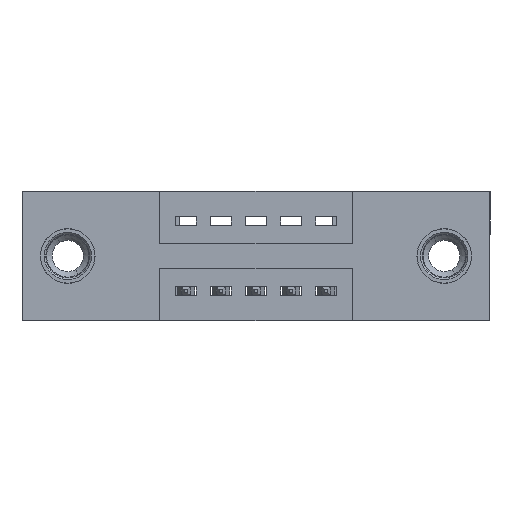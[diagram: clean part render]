
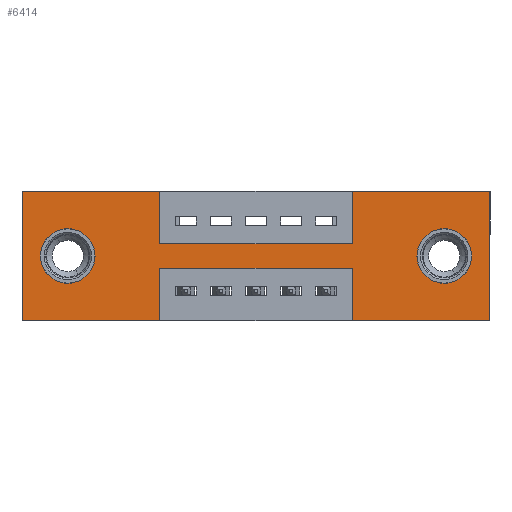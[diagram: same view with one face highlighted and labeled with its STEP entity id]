
A CAD part, front view. The second image highlights one B-rep face of the part: STEP entity #6414.
In plain terms, the highlighted planar face has unit normal (0, -1, 0).
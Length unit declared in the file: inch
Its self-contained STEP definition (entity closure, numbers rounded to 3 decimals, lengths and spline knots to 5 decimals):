
#1 = EDGE_CURVE ( 'NONE', #5231, #4757, #5627, .T. ) ;
#156 = CARTESIAN_POINT ( 'NONE',  ( 1.335, 0., 0. ) ) ;
#190 = VECTOR ( 'NONE', #808, 39.37008 ) ;
#221 = DIRECTION ( 'NONE',  ( 1., 0., 0. ) ) ;
#294 = ORIENTED_EDGE ( 'NONE', *, *, #10173, .F. ) ;
#348 = DIRECTION ( 'NONE',  ( 0., 0., -1. ) ) ;
#634 = CARTESIAN_POINT ( 'NONE',  ( 0.9425, 0., -0.37 ) ) ;
#799 = ORIENTED_EDGE ( 'NONE', *, *, #4436, .T. ) ;
#808 = DIRECTION ( 'NONE',  ( -1., 0., 0. ) ) ;
#852 = DIRECTION ( 'NONE',  ( 1., 0., 0. ) ) ;
#879 = VECTOR ( 'NONE', #11801, 39.37008 ) ;
#882 = VERTEX_POINT ( 'NONE', #13210 ) ;
#1131 = ORIENTED_EDGE ( 'NONE', *, *, #8458, .F. ) ;
#1225 = VERTEX_POINT ( 'NONE', #11011 ) ;
#1478 = EDGE_CURVE ( 'NONE', #882, #12345, #8987, .T. ) ;
#1762 = DIRECTION ( 'NONE',  ( 0., 1., 0. ) ) ;
#1803 = VECTOR ( 'NONE', #9469, 39.37008 ) ;
#1930 = CIRCLE ( 'NONE', #8723, 0.078 ) ;
#1942 = VERTEX_POINT ( 'NONE', #3458 ) ;
#2013 = LINE ( 'NONE', #5888, #190 ) ;
#2063 = CARTESIAN_POINT ( 'NONE',  ( 0.3925, 0., -0.15 ) ) ;
#2175 = EDGE_CURVE ( 'NONE', #4079, #2269, #10104, .T. ) ;
#2202 = CARTESIAN_POINT ( 'NONE',  ( 0.3925, 0., 0. ) ) ;
#2213 = LINE ( 'NONE', #11607, #879 ) ;
#2269 = VERTEX_POINT ( 'NONE', #2063 ) ;
#2405 = DIRECTION ( 'NONE',  ( 0., 1., 0. ) ) ;
#2603 = DIRECTION ( 'NONE',  ( 0., 0., 1. ) ) ;
#2610 = LINE ( 'NONE', #156, #4736 ) ;
#2804 = CARTESIAN_POINT ( 'NONE',  ( 1.205, 0., -0.263 ) ) ;
#2836 = DIRECTION ( 'NONE',  ( 0., 1., 0. ) ) ;
#2844 = ORIENTED_EDGE ( 'NONE', *, *, #12134, .F. ) ;
#2877 = ORIENTED_EDGE ( 'NONE', *, *, #9994, .F. ) ;
#2954 = CIRCLE ( 'NONE', #8799, 0.078 ) ;
#3016 = EDGE_CURVE ( 'NONE', #12345, #882, #2954, .T. ) ;
#3038 = VERTEX_POINT ( 'NONE', #5098 ) ;
#3049 = DIRECTION ( 'NONE',  ( 1., 0., 0. ) ) ;
#3199 = LINE ( 'NONE', #12943, #9703 ) ;
#3251 = VECTOR ( 'NONE', #3366, 39.37008 ) ;
#3338 = DIRECTION ( 'NONE',  ( 0., 0., -1. ) ) ;
#3366 = DIRECTION ( 'NONE',  ( -1., 0., 0. ) ) ;
#3446 = VERTEX_POINT ( 'NONE', #5928 ) ;
#3458 = CARTESIAN_POINT ( 'NONE',  ( 1.205, 0., -0.107 ) ) ;
#3540 = VECTOR ( 'NONE', #11169, 39.37008 ) ;
#3643 = DIRECTION ( 'NONE',  ( 0., 0., -1. ) ) ;
#3817 = EDGE_LOOP ( 'NONE', ( #9071, #799 ) ) ;
#4062 = CARTESIAN_POINT ( 'NONE',  ( 0., 0., 0. ) ) ;
#4066 = EDGE_CURVE ( 'NONE', #4757, #4079, #6829, .T. ) ;
#4079 = VERTEX_POINT ( 'NONE', #6170 ) ;
#4179 = EDGE_CURVE ( 'NONE', #1942, #7464, #4877, .T. ) ;
#4324 = CARTESIAN_POINT ( 'NONE',  ( 0.3925, 0., -0.37 ) ) ;
#4436 = EDGE_CURVE ( 'NONE', #7464, #1942, #1930, .T. ) ;
#4492 = VECTOR ( 'NONE', #6639, 39.37008 ) ;
#4644 = CARTESIAN_POINT ( 'NONE',  ( 0., 0., 0. ) ) ;
#4697 = LINE ( 'NONE', #4644, #7109 ) ;
#4736 = VECTOR ( 'NONE', #3338, 39.37008 ) ;
#4757 = VERTEX_POINT ( 'NONE', #5470 ) ;
#4845 = LINE ( 'NONE', #4893, #3540 ) ;
#4856 = DIRECTION ( 'NONE',  ( 0., 0., 1. ) ) ;
#4877 = CIRCLE ( 'NONE', #9601, 0.078 ) ;
#4893 = CARTESIAN_POINT ( 'NONE',  ( 0.3925, 0., -0.37 ) ) ;
#5043 = VECTOR ( 'NONE', #3049, 39.37008 ) ;
#5067 = VERTEX_POINT ( 'NONE', #7814 ) ;
#5098 = CARTESIAN_POINT ( 'NONE',  ( 0.9425, 0., -0.37 ) ) ;
#5231 = VERTEX_POINT ( 'NONE', #7160 ) ;
#5272 = VERTEX_POINT ( 'NONE', #12498 ) ;
#5434 = CARTESIAN_POINT ( 'NONE',  ( 0.3925, 0., -0.22 ) ) ;
#5470 = CARTESIAN_POINT ( 'NONE',  ( 0., 0., 0. ) ) ;
#5618 = CARTESIAN_POINT ( 'NONE',  ( 0.13, 0., -0.185 ) ) ;
#5627 = LINE ( 'NONE', #6863, #4492 ) ;
#5759 = AXIS2_PLACEMENT_3D ( 'NONE', #5618, #10850, #2603 ) ;
#5772 = VERTEX_POINT ( 'NONE', #4324 ) ;
#5812 = EDGE_CURVE ( 'NONE', #9942, #5067, #2213, .T. ) ;
#5888 = CARTESIAN_POINT ( 'NONE',  ( 0., 0., -0.37 ) ) ;
#5928 = CARTESIAN_POINT ( 'NONE',  ( 0.9425, 0., -0.22 ) ) ;
#5950 = DIRECTION ( 'NONE',  ( 0., 0., -1. ) ) ;
#5993 = ORIENTED_EDGE ( 'NONE', *, *, #3016, .T. ) ;
#6170 = CARTESIAN_POINT ( 'NONE',  ( 0.3925, 0., 0. ) ) ;
#6239 = VERTEX_POINT ( 'NONE', #12690 ) ;
#6414 = ADVANCED_FACE ( 'NONE', ( #12539, #8442, #11675 ), #8826, .T. ) ;
#6609 = DIRECTION ( 'NONE',  ( 0., -1., 0. ) ) ;
#6639 = DIRECTION ( 'NONE',  ( 0., 0., 1. ) ) ;
#6801 = EDGE_LOOP ( 'NONE', ( #13529, #11722, #10774, #294, #1131, #2877, #13084, #2844, #10058, #8311, #10654, #8742 ) ) ;
#6829 = LINE ( 'NONE', #4062, #5043 ) ;
#6863 = CARTESIAN_POINT ( 'NONE',  ( 0., 0., 0. ) ) ;
#7082 = DIRECTION ( 'NONE',  ( 0., 0., 1. ) ) ;
#7109 = VECTOR ( 'NONE', #221, 39.37008 ) ;
#7110 = ORIENTED_EDGE ( 'NONE', *, *, #1478, .T. ) ;
#7160 = CARTESIAN_POINT ( 'NONE',  ( 0., 0., -0.37 ) ) ;
#7375 = CARTESIAN_POINT ( 'NONE',  ( 0.9425, 0., -0.15 ) ) ;
#7464 = VERTEX_POINT ( 'NONE', #2804 ) ;
#7613 = CARTESIAN_POINT ( 'NONE',  ( 1.205, 0., -0.185 ) ) ;
#7814 = CARTESIAN_POINT ( 'NONE',  ( 0.9425, 0., 0. ) ) ;
#7964 = LINE ( 'NONE', #5434, #3251 ) ;
#7991 = CARTESIAN_POINT ( 'NONE',  ( 0.13, 0., -0.185 ) ) ;
#8156 = EDGE_CURVE ( 'NONE', #3446, #5272, #7964, .T. ) ;
#8212 = CARTESIAN_POINT ( 'NONE',  ( 0.3925, 0., -0.15 ) ) ;
#8311 = ORIENTED_EDGE ( 'NONE', *, *, #4066, .F. ) ;
#8442 = FACE_BOUND ( 'NONE', #11724, .T. ) ;
#8458 = EDGE_CURVE ( 'NONE', #6239, #1225, #2610, .T. ) ;
#8723 = AXIS2_PLACEMENT_3D ( 'NONE', #9589, #2836, #5950 ) ;
#8742 = ORIENTED_EDGE ( 'NONE', *, *, #11865, .F. ) ;
#8799 = AXIS2_PLACEMENT_3D ( 'NONE', #7991, #1762, #7082 ) ;
#8826 = PLANE ( 'NONE',  #12055 ) ;
#8987 = CIRCLE ( 'NONE', #5759, 0.078 ) ;
#9071 = ORIENTED_EDGE ( 'NONE', *, *, #4179, .T. ) ;
#9469 = DIRECTION ( 'NONE',  ( 0., 0., -1. ) ) ;
#9589 = CARTESIAN_POINT ( 'NONE',  ( 1.205, 0., -0.185 ) ) ;
#9601 = AXIS2_PLACEMENT_3D ( 'NONE', #7613, #2405, #3643 ) ;
#9661 = VECTOR ( 'NONE', #852, 39.37008 ) ;
#9703 = VECTOR ( 'NONE', #9852, 39.37008 ) ;
#9852 = DIRECTION ( 'NONE',  ( -1., 0., 0. ) ) ;
#9883 = CARTESIAN_POINT ( 'NONE',  ( 0., 0., -0.37 ) ) ;
#9942 = VERTEX_POINT ( 'NONE', #7375 ) ;
#9992 = LINE ( 'NONE', #8212, #9661 ) ;
#9994 = EDGE_CURVE ( 'NONE', #5067, #6239, #4697, .T. ) ;
#10058 = ORIENTED_EDGE ( 'NONE', *, *, #2175, .F. ) ;
#10104 = LINE ( 'NONE', #2202, #1803 ) ;
#10159 = EDGE_CURVE ( 'NONE', #3038, #3446, #11640, .T. ) ;
#10173 = EDGE_CURVE ( 'NONE', #1225, #3038, #3199, .T. ) ;
#10232 = EDGE_CURVE ( 'NONE', #5272, #5772, #4845, .T. ) ;
#10654 = ORIENTED_EDGE ( 'NONE', *, *, #1, .F. ) ;
#10774 = ORIENTED_EDGE ( 'NONE', *, *, #10159, .F. ) ;
#10850 = DIRECTION ( 'NONE',  ( 0., 1., 0. ) ) ;
#10971 = CARTESIAN_POINT ( 'NONE',  ( 0.13, 0., -0.107 ) ) ;
#11011 = CARTESIAN_POINT ( 'NONE',  ( 1.335, 0., -0.37 ) ) ;
#11169 = DIRECTION ( 'NONE',  ( 0., 0., -1. ) ) ;
#11465 = VECTOR ( 'NONE', #4856, 39.37008 ) ;
#11607 = CARTESIAN_POINT ( 'NONE',  ( 0.9425, 0., 0. ) ) ;
#11640 = LINE ( 'NONE', #634, #11465 ) ;
#11675 = FACE_OUTER_BOUND ( 'NONE', #6801, .T. ) ;
#11722 = ORIENTED_EDGE ( 'NONE', *, *, #8156, .F. ) ;
#11724 = EDGE_LOOP ( 'NONE', ( #5993, #7110 ) ) ;
#11801 = DIRECTION ( 'NONE',  ( 0., 0., 1. ) ) ;
#11865 = EDGE_CURVE ( 'NONE', #5772, #5231, #2013, .T. ) ;
#12055 = AXIS2_PLACEMENT_3D ( 'NONE', #9883, #6609, #348 ) ;
#12134 = EDGE_CURVE ( 'NONE', #2269, #9942, #9992, .T. ) ;
#12345 = VERTEX_POINT ( 'NONE', #10971 ) ;
#12498 = CARTESIAN_POINT ( 'NONE',  ( 0.3925, 0., -0.22 ) ) ;
#12539 = FACE_BOUND ( 'NONE', #3817, .T. ) ;
#12690 = CARTESIAN_POINT ( 'NONE',  ( 1.335, 0., 0. ) ) ;
#12943 = CARTESIAN_POINT ( 'NONE',  ( 0., 0., -0.37 ) ) ;
#13084 = ORIENTED_EDGE ( 'NONE', *, *, #5812, .F. ) ;
#13210 = CARTESIAN_POINT ( 'NONE',  ( 0.13, 0., -0.263 ) ) ;
#13529 = ORIENTED_EDGE ( 'NONE', *, *, #10232, .F. ) ;
